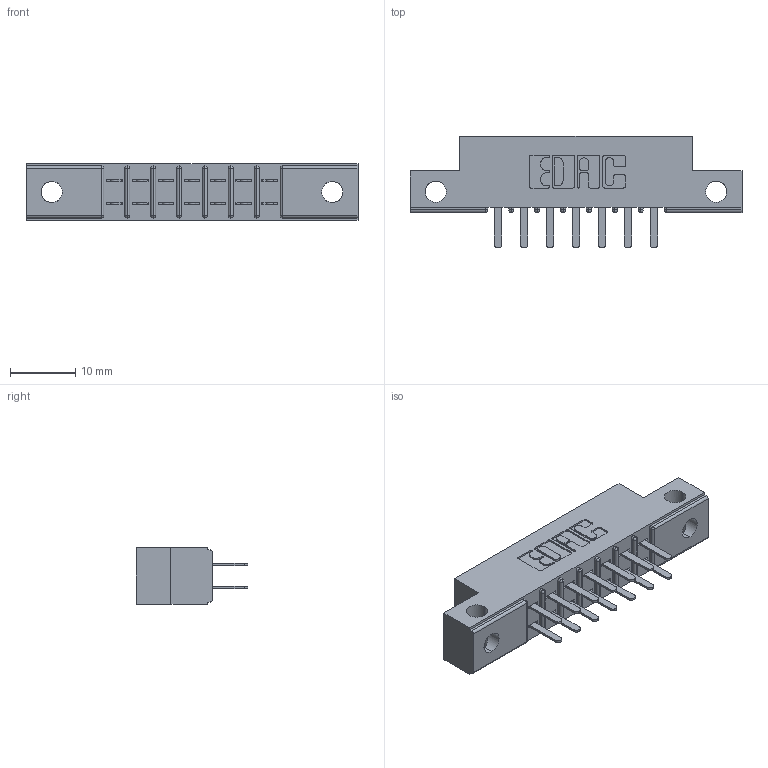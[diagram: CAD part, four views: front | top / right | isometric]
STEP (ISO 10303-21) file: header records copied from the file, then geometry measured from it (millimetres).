
FILE_DESCRIPTION (( 'STEP AP203' ), '1' );
FILE_NAME ('305-014-520-512.STEP', '2020-09-19T20:22:07', ( '' ), ( '' ), 'SwSTEP 2.0', 'SolidWorks 2020', '' );
FILE_SCHEMA (( 'CONFIG_CONTROL_DESIGN' ));
Length unit declared in the file: inch
Products named in the file (3): 305-290-001_520; 305-014-520-512; 305 Part_.128 Dia
Assembly tree (15 placements, depth 2):
  305-014-520-512
    305 Part_.128 Dia
    305-290-001_520  x14
Bounding box: 50.75 x 17.09 x 8.71 mm (x, y, z)
Volume: 2963.7 mm3; surface area: 4963 mm2
Topology: 15 solids, 15 shells, 772 faces, 2193 edges, 1418 vertices
Faces by surface type: plane 446, cylinder 298, sphere 28
Entity records: 12126 total; most frequent: CARTESIAN_POINT 2055, ORIENTED_EDGE 1990, DIRECTION 1955, EDGE_CURVE 995, VECTOR 751, LINE 751, VERTEX_POINT 638, AXIS2_PLACEMENT_3D 602
